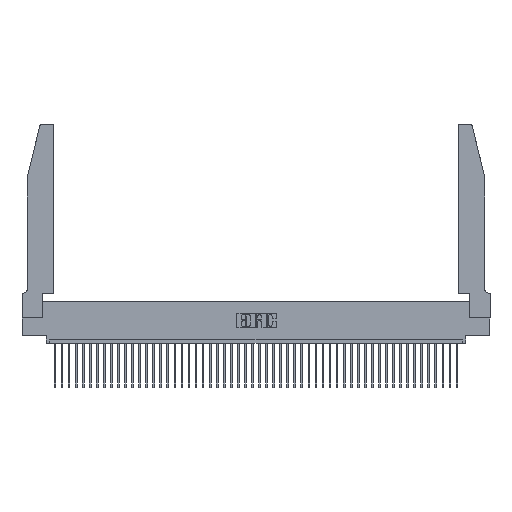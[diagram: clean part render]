
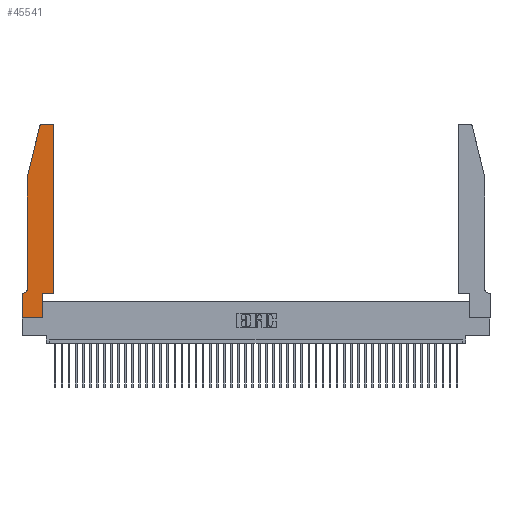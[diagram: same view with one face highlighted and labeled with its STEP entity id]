
A CAD part, top view. The second image highlights one B-rep face of the part: STEP entity #45541.
In plain terms, the highlighted planar face has unit normal (0, 0, 1).
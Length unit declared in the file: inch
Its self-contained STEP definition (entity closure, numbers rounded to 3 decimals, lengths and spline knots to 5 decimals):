
#47 = VERTEX_POINT ( 'NONE', #12227 ) ;
#77 = VERTEX_POINT ( 'NONE', #22445 ) ;
#173 = VECTOR ( 'NONE', #8768, 39.37008 ) ;
#519 = DIRECTION ( 'NONE',  ( 1., 0., 0. ) ) ;
#751 = DIRECTION ( 'NONE',  ( 0., 0., 1. ) ) ;
#858 = ORIENTED_EDGE ( 'NONE', *, *, #23044, .T. ) ;
#1481 = VERTEX_POINT ( 'NONE', #35764 ) ;
#1495 = VERTEX_POINT ( 'NONE', #14154 ) ;
#2004 = DIRECTION ( 'NONE',  ( 0., -1., 0. ) ) ;
#2350 = ORIENTED_EDGE ( 'NONE', *, *, #34553, .T. ) ;
#2996 = DIRECTION ( 'NONE',  ( -1., 0., 0. ) ) ;
#3665 = CARTESIAN_POINT ( 'NONE',  ( 0.4505, 0.35, 0.37 ) ) ;
#3769 = DIRECTION ( 'NONE',  ( 0., 0., -1. ) ) ;
#4125 = ORIENTED_EDGE ( 'NONE', *, *, #43028, .T. ) ;
#4400 = EDGE_CURVE ( 'NONE', #77, #47, #7478, .T. ) ;
#5144 = LINE ( 'NONE', #18685, #20294 ) ;
#5172 = CARTESIAN_POINT ( 'NONE',  ( 0.4505, 0.35, 0.37 ) ) ;
#5409 = EDGE_CURVE ( 'NONE', #1481, #44656, #43245, .T. ) ;
#5566 = LINE ( 'NONE', #29325, #20123 ) ;
#5765 = DIRECTION ( 'NONE',  ( -1., 0., 0. ) ) ;
#5819 = LINE ( 'NONE', #5172, #173 ) ;
#6031 = FACE_OUTER_BOUND ( 'NONE', #21949, .T. ) ;
#6258 = DIRECTION ( 'NONE',  ( -0.239, -0.971, 0. ) ) ;
#7129 = VERTEX_POINT ( 'NONE', #39017 ) ;
#7478 = CIRCLE ( 'NONE', #28989, 0.07 ) ;
#8768 = DIRECTION ( 'NONE',  ( 0., 1., 0. ) ) ;
#8845 = DIRECTION ( 'NONE',  ( 1., 0., 0. ) ) ;
#9015 = CARTESIAN_POINT ( 'NONE',  ( 0., 0., 0.37 ) ) ;
#10163 = ORIENTED_EDGE ( 'NONE', *, *, #29083, .T. ) ;
#10457 = EDGE_CURVE ( 'NONE', #38028, #1481, #37888, .T. ) ;
#10860 = ORIENTED_EDGE ( 'NONE', *, *, #43231, .T. ) ;
#10986 = DIRECTION ( 'NONE',  ( 1., 0., 0. ) ) ;
#11004 = CIRCLE ( 'NONE', #25436, 0.03 ) ;
#12227 = CARTESIAN_POINT ( 'NONE',  ( 0.0055, 0.35, 0.37 ) ) ;
#13224 = LINE ( 'NONE', #9015, #30716 ) ;
#13913 = DIRECTION ( 'NONE',  ( 0., 1., 0. ) ) ;
#14154 = CARTESIAN_POINT ( 'NONE',  ( 0.0755, 2., 0.37 ) ) ;
#15385 = CARTESIAN_POINT ( 'NONE',  ( 0.4205, 2.75, 0.37 ) ) ;
#16875 = LINE ( 'NONE', #39004, #46086 ) ;
#17257 = DIRECTION ( 'NONE',  ( 1., 0., 0. ) ) ;
#18482 = CARTESIAN_POINT ( 'NONE',  ( 0.4205, 2.72, 0.37 ) ) ;
#18672 = ORIENTED_EDGE ( 'NONE', *, *, #45633, .T. ) ;
#18685 = CARTESIAN_POINT ( 'NONE',  ( 0., 0., 0.37 ) ) ;
#18768 = VERTEX_POINT ( 'NONE', #28275 ) ;
#19015 = PLANE ( 'NONE',  #25616 ) ;
#20123 = VECTOR ( 'NONE', #21890, 39.37008 ) ;
#20294 = VECTOR ( 'NONE', #519, 39.37008 ) ;
#21890 = DIRECTION ( 'NONE',  ( 0., -1., 0. ) ) ;
#21949 = EDGE_LOOP ( 'NONE', ( #10860, #858, #26547, #22178, #45514, #39684, #18672, #4125, #33337, #39453, #10163, #2350 ) ) ;
#22038 = DIRECTION ( 'NONE',  ( 1., 0., 0. ) ) ;
#22178 = ORIENTED_EDGE ( 'NONE', *, *, #44718, .T. ) ;
#22445 = CARTESIAN_POINT ( 'NONE',  ( 0.0755, 0.42, 0.37 ) ) ;
#22653 = EDGE_CURVE ( 'NONE', #39547, #1495, #23354, .T. ) ;
#22791 = CARTESIAN_POINT ( 'NONE',  ( 0., 0.35, 0.37 ) ) ;
#23044 = EDGE_CURVE ( 'NONE', #18768, #39547, #24485, .T. ) ;
#23354 = LINE ( 'NONE', #45589, #44670 ) ;
#23855 = VECTOR ( 'NONE', #13913, 39.37008 ) ;
#24029 = VERTEX_POINT ( 'NONE', #15385 ) ;
#24392 = CARTESIAN_POINT ( 'NONE',  ( 0.2865, 0.35, 0.37 ) ) ;
#24485 = CIRCLE ( 'NONE', #24864, 0.03 ) ;
#24864 = AXIS2_PLACEMENT_3D ( 'NONE', #43802, #751, #22038 ) ;
#25436 = AXIS2_PLACEMENT_3D ( 'NONE', #18482, #28148, #10986 ) ;
#25616 = AXIS2_PLACEMENT_3D ( 'NONE', #44234, #30382, #8845 ) ;
#26162 = DIRECTION ( 'NONE',  ( -1., 0., 0. ) ) ;
#26547 = ORIENTED_EDGE ( 'NONE', *, *, #22653, .T. ) ;
#27122 = CARTESIAN_POINT ( 'NONE',  ( 0.0755, 0.35, 0.37 ) ) ;
#27178 = LINE ( 'NONE', #27122, #42779 ) ;
#27499 = CARTESIAN_POINT ( 'NONE',  ( 0., 0., 0.37 ) ) ;
#28148 = DIRECTION ( 'NONE',  ( 0., 0., 1. ) ) ;
#28235 = VECTOR ( 'NONE', #17257, 39.37008 ) ;
#28275 = CARTESIAN_POINT ( 'NONE',  ( 0.284, 2.75, 0.37 ) ) ;
#28516 = EDGE_CURVE ( 'NONE', #47, #40954, #27178, .T. ) ;
#28989 = AXIS2_PLACEMENT_3D ( 'NONE', #34998, #3769, #26162 ) ;
#29083 = EDGE_CURVE ( 'NONE', #44656, #7129, #5819, .T. ) ;
#29325 = CARTESIAN_POINT ( 'NONE',  ( 0.0755, 2., 0.37 ) ) ;
#30382 = DIRECTION ( 'NONE',  ( 0., 0., 1. ) ) ;
#30716 = VECTOR ( 'NONE', #2004, 39.37008 ) ;
#33337 = ORIENTED_EDGE ( 'NONE', *, *, #10457, .T. ) ;
#34553 = EDGE_CURVE ( 'NONE', #7129, #24029, #11004, .T. ) ;
#34998 = CARTESIAN_POINT ( 'NONE',  ( 0.0055, 0.42, 0.37 ) ) ;
#35764 = CARTESIAN_POINT ( 'NONE',  ( 0.2865, 0.35, 0.37 ) ) ;
#36343 = VERTEX_POINT ( 'NONE', #27499 ) ;
#37888 = LINE ( 'NONE', #24392, #23855 ) ;
#38028 = VERTEX_POINT ( 'NONE', #39240 ) ;
#39004 = CARTESIAN_POINT ( 'NONE',  ( 0.2605, 2.75, 0.37 ) ) ;
#39017 = CARTESIAN_POINT ( 'NONE',  ( 0.4505, 2.72, 0.37 ) ) ;
#39240 = CARTESIAN_POINT ( 'NONE',  ( 0.2865, 0., 0.37 ) ) ;
#39453 = ORIENTED_EDGE ( 'NONE', *, *, #5409, .T. ) ;
#39547 = VERTEX_POINT ( 'NONE', #45902 ) ;
#39684 = ORIENTED_EDGE ( 'NONE', *, *, #28516, .T. ) ;
#40954 = VERTEX_POINT ( 'NONE', #22791 ) ;
#42779 = VECTOR ( 'NONE', #5765, 39.37008 ) ;
#43028 = EDGE_CURVE ( 'NONE', #36343, #38028, #5144, .T. ) ;
#43231 = EDGE_CURVE ( 'NONE', #24029, #18768, #16875, .T. ) ;
#43245 = LINE ( 'NONE', #3665, #28235 ) ;
#43802 = CARTESIAN_POINT ( 'NONE',  ( 0.284, 2.72, 0.37 ) ) ;
#44234 = CARTESIAN_POINT ( 'NONE',  ( 0., 0.35, 0.37 ) ) ;
#44656 = VERTEX_POINT ( 'NONE', #46405 ) ;
#44670 = VECTOR ( 'NONE', #6258, 39.37008 ) ;
#44718 = EDGE_CURVE ( 'NONE', #1495, #77, #5566, .T. ) ;
#45514 = ORIENTED_EDGE ( 'NONE', *, *, #4400, .T. ) ;
#45541 = ADVANCED_FACE ( 'NONE', ( #6031 ), #19015, .T. ) ;
#45589 = CARTESIAN_POINT ( 'NONE',  ( 0.0755, 2., 0.37 ) ) ;
#45633 = EDGE_CURVE ( 'NONE', #40954, #36343, #13224, .T. ) ;
#45902 = CARTESIAN_POINT ( 'NONE',  ( 0.25487, 2.72718, 0.37 ) ) ;
#46086 = VECTOR ( 'NONE', #2996, 39.37008 ) ;
#46405 = CARTESIAN_POINT ( 'NONE',  ( 0.4505, 0.35, 0.37 ) ) ;
